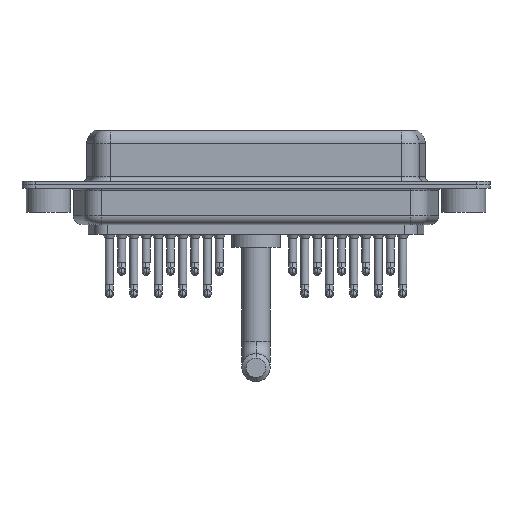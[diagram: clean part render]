
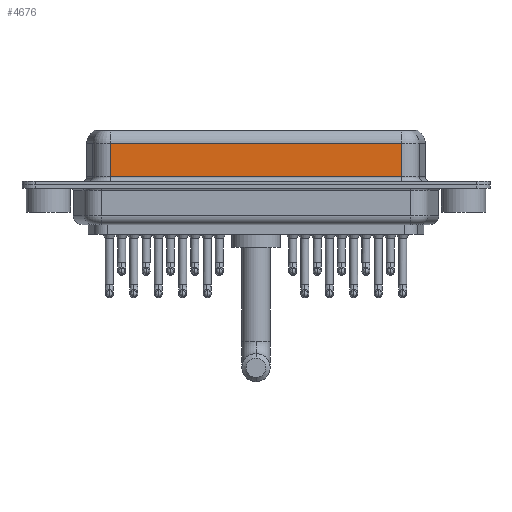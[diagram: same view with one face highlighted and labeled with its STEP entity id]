
A CAD part, front view. The second image highlights one B-rep face of the part: STEP entity #4676.
In plain terms, the highlighted planar face has unit normal (0, -1, 0).
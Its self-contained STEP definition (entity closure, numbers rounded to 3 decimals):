
#352 = VECTOR ( 'NONE', #15660, 1000. ) ;
#499 = VECTOR ( 'NONE', #20528, 1000. ) ;
#828 = VERTEX_POINT ( 'NONE', #12760 ) ;
#3156 = FACE_OUTER_BOUND ( 'NONE', #16429, .T. ) ;
#3594 = ORIENTED_EDGE ( 'NONE', *, *, #14183, .T. ) ;
#4676 = ADVANCED_FACE ( 'NONE', ( #3156 ), #8210, .F. ) ;
#4755 = LINE ( 'NONE', #8190, #499 ) ;
#6303 = CARTESIAN_POINT ( 'NONE',  ( 40.037, -3.95, 0.9 ) ) ;
#6355 = EDGE_CURVE ( 'NONE', #8389, #20446, #4755, .T. ) ;
#8190 = CARTESIAN_POINT ( 'NONE',  ( 40.037, -3.95, 6.4 ) ) ;
#8210 = PLANE ( 'NONE',  #14307 ) ;
#8389 = VERTEX_POINT ( 'NONE', #21704 ) ;
#8433 = CARTESIAN_POINT ( 'NONE',  ( 40.037, -3.95, 4.65 ) ) ;
#9400 = VERTEX_POINT ( 'NONE', #15421 ) ;
#9797 = CARTESIAN_POINT ( 'NONE',  ( 40.037, -3.95, 6.4 ) ) ;
#10316 = EDGE_CURVE ( 'NONE', #828, #9400, #11140, .T. ) ;
#11140 = LINE ( 'NONE', #18006, #14220 ) ;
#12460 = LINE ( 'NONE', #19327, #352 ) ;
#12760 = CARTESIAN_POINT ( 'NONE',  ( 7.013, -3.95, 4.65 ) ) ;
#12963 = ORIENTED_EDGE ( 'NONE', *, *, #6355, .F. ) ;
#14183 = EDGE_CURVE ( 'NONE', #9400, #20446, #12460, .T. ) ;
#14220 = VECTOR ( 'NONE', #21224, 1000. ) ;
#14307 = AXIS2_PLACEMENT_3D ( 'NONE', #9797, #18826, #16747 ) ;
#15387 = DIRECTION ( 'NONE',  ( -1., 0., 0. ) ) ;
#15421 = CARTESIAN_POINT ( 'NONE',  ( 7.013, -3.95, 0.9 ) ) ;
#15660 = DIRECTION ( 'NONE',  ( 1., 0., 0. ) ) ;
#16429 = EDGE_LOOP ( 'NONE', ( #12963, #18293, #20109, #3594 ) ) ;
#16747 = DIRECTION ( 'NONE',  ( 0., 0., 1. ) ) ;
#17844 = VECTOR ( 'NONE', #15387, 1000. ) ;
#18006 = CARTESIAN_POINT ( 'NONE',  ( 7.013, -3.95, 6.4 ) ) ;
#18293 = ORIENTED_EDGE ( 'NONE', *, *, #19936, .T. ) ;
#18826 = DIRECTION ( 'NONE',  ( 0., 1., 0. ) ) ;
#19327 = CARTESIAN_POINT ( 'NONE',  ( 40.037, -3.95, 0.9 ) ) ;
#19936 = EDGE_CURVE ( 'NONE', #8389, #828, #20884, .T. ) ;
#20109 = ORIENTED_EDGE ( 'NONE', *, *, #10316, .T. ) ;
#20446 = VERTEX_POINT ( 'NONE', #6303 ) ;
#20528 = DIRECTION ( 'NONE',  ( 0., 0., -1. ) ) ;
#20884 = LINE ( 'NONE', #8433, #17844 ) ;
#21224 = DIRECTION ( 'NONE',  ( 0., 0., -1. ) ) ;
#21704 = CARTESIAN_POINT ( 'NONE',  ( 40.037, -3.95, 4.65 ) ) ;
